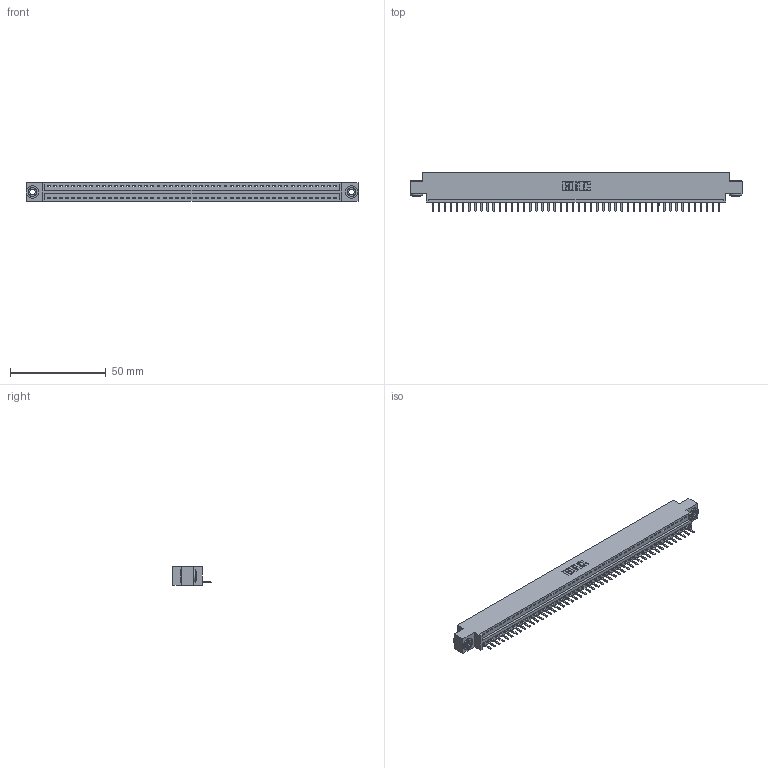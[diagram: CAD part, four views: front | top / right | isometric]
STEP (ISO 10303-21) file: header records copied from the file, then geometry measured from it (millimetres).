
FILE_DESCRIPTION (( 'STEP AP203' ), '1' );
FILE_NAME ('396-048-520-603.STEP', '2018-09-07T11:44:28', ( '' ), ( '' ), 'SwSTEP 2.0', 'SolidWorks 2016', '' );
FILE_SCHEMA (( 'CONFIG_CONTROL_DESIGN' ));
Length unit declared in the file: inch
Products named in the file (4): 345-292-001_345-293-120; 345-250-002_345-250-002-102; 396-048-520-603; 346 Part_0.170 Offset - 0.156 Dia-TH
Assembly tree (51 placements, depth 2):
  396-048-520-603
    346 Part_0.170 Offset - 0.156 Dia-TH
    345-292-001_345-293-120  x48
    345-250-002_345-250-002-102  x2
Bounding box: 172.97 x 20.02 x 9.4 mm (x, y, z)
Volume: 16325.5 mm3; surface area: 20388.1 mm2
Topology: 51 solids, 51 shells, 3140 faces, 9249 edges, 6034 vertices
Faces by surface type: plane 2106, cylinder 1026, cone 8
Entity records: 29878 total; most frequent: CARTESIAN_POINT 5111, ORIENTED_EDGE 5074, DIRECTION 4519, EDGE_CURVE 2537, LINE 2185, VECTOR 2185, VERTEX_POINT 1686, AXIS2_PLACEMENT_3D 1167
